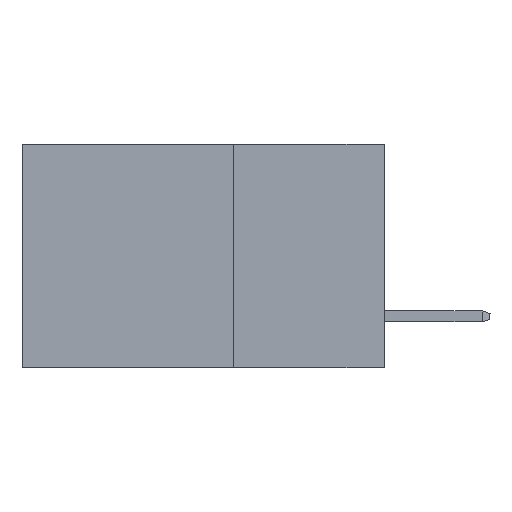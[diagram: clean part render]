
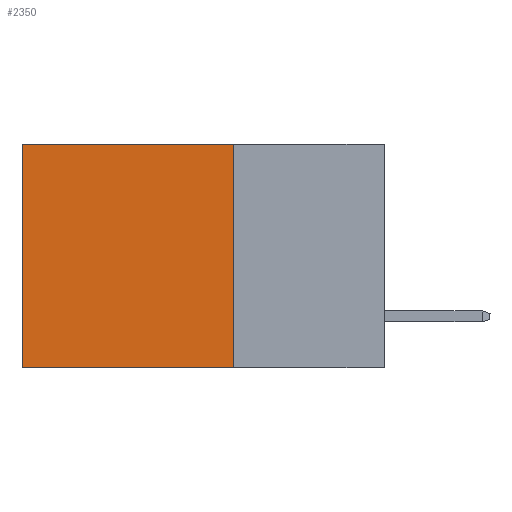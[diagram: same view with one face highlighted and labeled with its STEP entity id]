
A CAD part, left-side view. The second image highlights one B-rep face of the part: STEP entity #2350.
In plain terms, the highlighted planar face has unit normal (-1, 0, 0).
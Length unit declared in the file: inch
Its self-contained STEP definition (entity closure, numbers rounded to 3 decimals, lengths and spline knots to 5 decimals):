
#764 = DIRECTION ( 'NONE',  ( 0., 1., 0. ) ) ;
#882 = LINE ( 'NONE', #1674, #9558 ) ;
#1117 = ORIENTED_EDGE ( 'NONE', *, *, #4752, .T. ) ;
#1546 = CARTESIAN_POINT ( 'NONE',  ( 0.2615, 0.25, -0.37 ) ) ;
#1674 = CARTESIAN_POINT ( 'NONE',  ( 0.2615, 0.25, -0.37 ) ) ;
#1877 = CARTESIAN_POINT ( 'NONE',  ( 0.2615, 0.6, -0.37 ) ) ;
#2176 = VERTEX_POINT ( 'NONE', #10141 ) ;
#2350 = ADVANCED_FACE ( 'NONE', ( #5888 ), #5106, .F. ) ;
#3033 = ORIENTED_EDGE ( 'NONE', *, *, #11766, .F. ) ;
#3846 = DIRECTION ( 'NONE',  ( 0., 0., -1. ) ) ;
#4211 = EDGE_LOOP ( 'NONE', ( #4438, #6032, #3033, #1117 ) ) ;
#4294 = CARTESIAN_POINT ( 'NONE',  ( 0.2615, 0.6, 0. ) ) ;
#4438 = ORIENTED_EDGE ( 'NONE', *, *, #9114, .T. ) ;
#4752 = EDGE_CURVE ( 'NONE', #7511, #11603, #7919, .T. ) ;
#4785 = CARTESIAN_POINT ( 'NONE',  ( 0.2615, 0.6, -0.37 ) ) ;
#5106 = PLANE ( 'NONE',  #9613 ) ;
#5223 = CARTESIAN_POINT ( 'NONE',  ( 0.2615, 0.25, 0. ) ) ;
#5888 = FACE_OUTER_BOUND ( 'NONE', #4211, .T. ) ;
#6032 = ORIENTED_EDGE ( 'NONE', *, *, #10295, .F. ) ;
#6520 = CARTESIAN_POINT ( 'NONE',  ( 0.2615, 0.25, -0.37 ) ) ;
#7481 = CARTESIAN_POINT ( 'NONE',  ( 0.2615, 0.25, 0. ) ) ;
#7511 = VERTEX_POINT ( 'NONE', #7481 ) ;
#7919 = LINE ( 'NONE', #5223, #11342 ) ;
#8000 = VECTOR ( 'NONE', #10305, 39.37008 ) ;
#8204 = DIRECTION ( 'NONE',  ( 0., 1., 0. ) ) ;
#8739 = DIRECTION ( 'NONE',  ( 1., 0., 0. ) ) ;
#8800 = DIRECTION ( 'NONE',  ( 0., 0., -1. ) ) ;
#9114 = EDGE_CURVE ( 'NONE', #11603, #10882, #11184, .T. ) ;
#9466 = LINE ( 'NONE', #6520, #9978 ) ;
#9558 = VECTOR ( 'NONE', #8204, 39.37008 ) ;
#9613 = AXIS2_PLACEMENT_3D ( 'NONE', #1546, #8739, #8800 ) ;
#9978 = VECTOR ( 'NONE', #3846, 39.37008 ) ;
#10141 = CARTESIAN_POINT ( 'NONE',  ( 0.2615, 0.25, -0.37 ) ) ;
#10295 = EDGE_CURVE ( 'NONE', #2176, #10882, #882, .T. ) ;
#10305 = DIRECTION ( 'NONE',  ( 0., 0., -1. ) ) ;
#10882 = VERTEX_POINT ( 'NONE', #1877 ) ;
#11184 = LINE ( 'NONE', #4785, #8000 ) ;
#11342 = VECTOR ( 'NONE', #764, 39.37008 ) ;
#11603 = VERTEX_POINT ( 'NONE', #4294 ) ;
#11766 = EDGE_CURVE ( 'NONE', #7511, #2176, #9466, .T. ) ;
